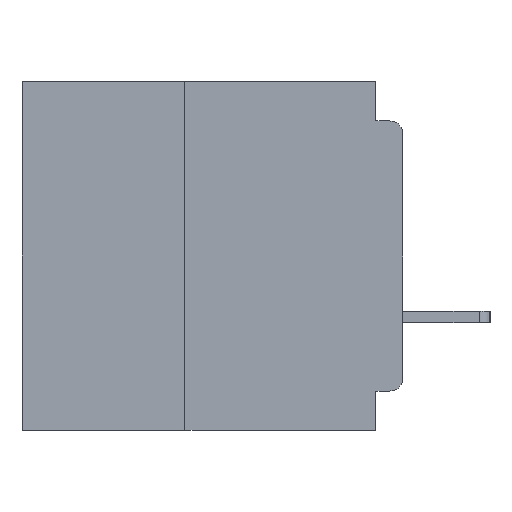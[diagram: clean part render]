
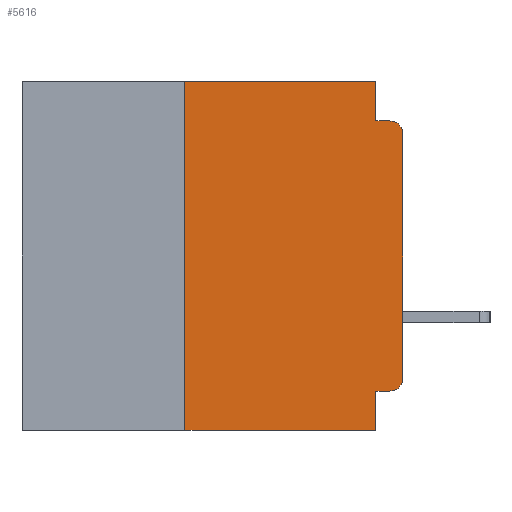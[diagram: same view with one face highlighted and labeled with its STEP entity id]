
A CAD part, left-side view. The second image highlights one B-rep face of the part: STEP entity #5616.
In plain terms, the highlighted planar face has unit normal (-1, 0, 0).
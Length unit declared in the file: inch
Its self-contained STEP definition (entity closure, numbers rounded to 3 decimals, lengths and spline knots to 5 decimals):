
#1761 = CARTESIAN_POINT ( 'NONE',  ( 0., 0., 0. ) ) ;
#2888 = VERTEX_POINT ( 'NONE', #36481 ) ;
#3490 = CARTESIAN_POINT ( 'NONE',  ( 0., 0.031, 0. ) ) ;
#3509 = DIRECTION ( 'NONE',  ( 0., -1., 0. ) ) ;
#3579 = EDGE_LOOP ( 'NONE', ( #4691, #5060, #16020, #11120, #11167, #25851, #38337, #17701, #5599, #17743 ) ) ;
#4691 = ORIENTED_EDGE ( 'NONE', *, *, #14274, .T. ) ;
#5060 = ORIENTED_EDGE ( 'NONE', *, *, #33131, .T. ) ;
#5336 = DIRECTION ( 'NONE',  ( 0., 0., 1. ) ) ;
#5599 = ORIENTED_EDGE ( 'NONE', *, *, #11302, .F. ) ;
#5616 = ADVANCED_FACE ( 'NONE', ( #32130 ), #20864, .F. ) ;
#6138 = DIRECTION ( 'NONE',  ( 0., 0., -1. ) ) ;
#6646 = CARTESIAN_POINT ( 'NONE',  ( 0., 0.031, -0.4 ) ) ;
#6969 = AXIS2_PLACEMENT_3D ( 'NONE', #11452, #35742, #14973 ) ;
#7050 = DIRECTION ( 'NONE',  ( 0., 0., -1. ) ) ;
#8022 = EDGE_CURVE ( 'NONE', #11762, #12928, #39513, .T. ) ;
#8266 = EDGE_CURVE ( 'NONE', #20146, #2888, #27508, .T. ) ;
#8703 = VECTOR ( 'NONE', #5336, 39.37008 ) ;
#9780 = EDGE_CURVE ( 'NONE', #14202, #37679, #37752, .T. ) ;
#11120 = ORIENTED_EDGE ( 'NONE', *, *, #40997, .F. ) ;
#11167 = ORIENTED_EDGE ( 'NONE', *, *, #12038, .F. ) ;
#11247 = DIRECTION ( 'NONE',  ( 0., 0., -1. ) ) ;
#11257 = LINE ( 'NONE', #18575, #28663 ) ;
#11302 = EDGE_CURVE ( 'NONE', #14202, #20146, #11257, .T. ) ;
#11303 = DIRECTION ( 'NONE',  ( -1., 0., 0. ) ) ;
#11363 = CARTESIAN_POINT ( 'NONE',  ( 0., 0.015, -0.34 ) ) ;
#11452 = CARTESIAN_POINT ( 'NONE',  ( 0., 0.015, -0.06 ) ) ;
#11762 = VERTEX_POINT ( 'NONE', #34919 ) ;
#12032 = DIRECTION ( 'NONE',  ( 0., -1., 0. ) ) ;
#12038 = EDGE_CURVE ( 'NONE', #30585, #30056, #25886, .T. ) ;
#12385 = CARTESIAN_POINT ( 'NONE',  ( 0., 0., -0.045 ) ) ;
#12928 = VERTEX_POINT ( 'NONE', #16627 ) ;
#13069 = EDGE_CURVE ( 'NONE', #37670, #2888, #18171, .T. ) ;
#14202 = VERTEX_POINT ( 'NONE', #25700 ) ;
#14274 = EDGE_CURVE ( 'NONE', #37679, #37973, #36480, .T. ) ;
#14973 = DIRECTION ( 'NONE',  ( 0., 0., -1. ) ) ;
#15473 = VECTOR ( 'NONE', #7050, 39.37008 ) ;
#15674 = CARTESIAN_POINT ( 'NONE',  ( 0., 0.25, -0.4 ) ) ;
#15768 = CARTESIAN_POINT ( 'NONE',  ( 0., 0., -0.34 ) ) ;
#16020 = ORIENTED_EDGE ( 'NONE', *, *, #8022, .F. ) ;
#16627 = CARTESIAN_POINT ( 'NONE',  ( 0., 0.015, -0.045 ) ) ;
#16973 = AXIS2_PLACEMENT_3D ( 'NONE', #20910, #21214, #20567 ) ;
#17701 = ORIENTED_EDGE ( 'NONE', *, *, #8266, .F. ) ;
#17742 = VECTOR ( 'NONE', #25977, 39.37008 ) ;
#17743 = ORIENTED_EDGE ( 'NONE', *, *, #9780, .T. ) ;
#18082 = AXIS2_PLACEMENT_3D ( 'NONE', #11363, #11303, #11247 ) ;
#18171 = LINE ( 'NONE', #31371, #35514 ) ;
#18575 = CARTESIAN_POINT ( 'NONE',  ( 0., 0., -0.355 ) ) ;
#20146 = VERTEX_POINT ( 'NONE', #24992 ) ;
#20567 = DIRECTION ( 'NONE',  ( 0., 0., -1. ) ) ;
#20864 = PLANE ( 'NONE',  #16973 ) ;
#20910 = CARTESIAN_POINT ( 'NONE',  ( 0., 0.437, 0. ) ) ;
#21214 = DIRECTION ( 'NONE',  ( 1., 0., 0. ) ) ;
#22759 = CARTESIAN_POINT ( 'NONE',  ( 0., 0.25, -0.4 ) ) ;
#23657 = CIRCLE ( 'NONE', #6969, 0.015 ) ;
#24992 = CARTESIAN_POINT ( 'NONE',  ( 0., 0.031, -0.355 ) ) ;
#25583 = DIRECTION ( 'NONE',  ( 0., 1., 0. ) ) ;
#25700 = CARTESIAN_POINT ( 'NONE',  ( 0., 0.015, -0.355 ) ) ;
#25851 = ORIENTED_EDGE ( 'NONE', *, *, #29350, .F. ) ;
#25886 = LINE ( 'NONE', #29469, #17742 ) ;
#25977 = DIRECTION ( 'NONE',  ( 0., -1., 0. ) ) ;
#27508 = LINE ( 'NONE', #6646, #44943 ) ;
#28082 = VECTOR ( 'NONE', #12032, 39.37008 ) ;
#28663 = VECTOR ( 'NONE', #25583, 39.37008 ) ;
#28914 = LINE ( 'NONE', #15674, #37034 ) ;
#29350 = EDGE_CURVE ( 'NONE', #37670, #30585, #28914, .T. ) ;
#29469 = CARTESIAN_POINT ( 'NONE',  ( 0., 0.437, 0. ) ) ;
#30056 = VERTEX_POINT ( 'NONE', #43532 ) ;
#30585 = VERTEX_POINT ( 'NONE', #35716 ) ;
#31371 = CARTESIAN_POINT ( 'NONE',  ( 0., 0.437, -0.4 ) ) ;
#32130 = FACE_OUTER_BOUND ( 'NONE', #3579, .T. ) ;
#32983 = DIRECTION ( 'NONE',  ( 0., 0., 1. ) ) ;
#33131 = EDGE_CURVE ( 'NONE', #37973, #12928, #23657, .T. ) ;
#33928 = LINE ( 'NONE', #3490, #15473 ) ;
#34919 = CARTESIAN_POINT ( 'NONE',  ( 0., 0.031, -0.045 ) ) ;
#35514 = VECTOR ( 'NONE', #3509, 39.37008 ) ;
#35716 = CARTESIAN_POINT ( 'NONE',  ( 0., 0.25, 0. ) ) ;
#35742 = DIRECTION ( 'NONE',  ( -1., 0., 0. ) ) ;
#36480 = LINE ( 'NONE', #1761, #8703 ) ;
#36481 = CARTESIAN_POINT ( 'NONE',  ( 0., 0.031, -0.4 ) ) ;
#37034 = VECTOR ( 'NONE', #32983, 39.37008 ) ;
#37670 = VERTEX_POINT ( 'NONE', #22759 ) ;
#37679 = VERTEX_POINT ( 'NONE', #15768 ) ;
#37752 = CIRCLE ( 'NONE', #18082, 0.015 ) ;
#37973 = VERTEX_POINT ( 'NONE', #41723 ) ;
#38337 = ORIENTED_EDGE ( 'NONE', *, *, #13069, .T. ) ;
#39513 = LINE ( 'NONE', #12385, #28082 ) ;
#40997 = EDGE_CURVE ( 'NONE', #30056, #11762, #33928, .T. ) ;
#41723 = CARTESIAN_POINT ( 'NONE',  ( 0., 0., -0.06 ) ) ;
#43532 = CARTESIAN_POINT ( 'NONE',  ( 0., 0.031, 0. ) ) ;
#44943 = VECTOR ( 'NONE', #6138, 39.37008 ) ;
